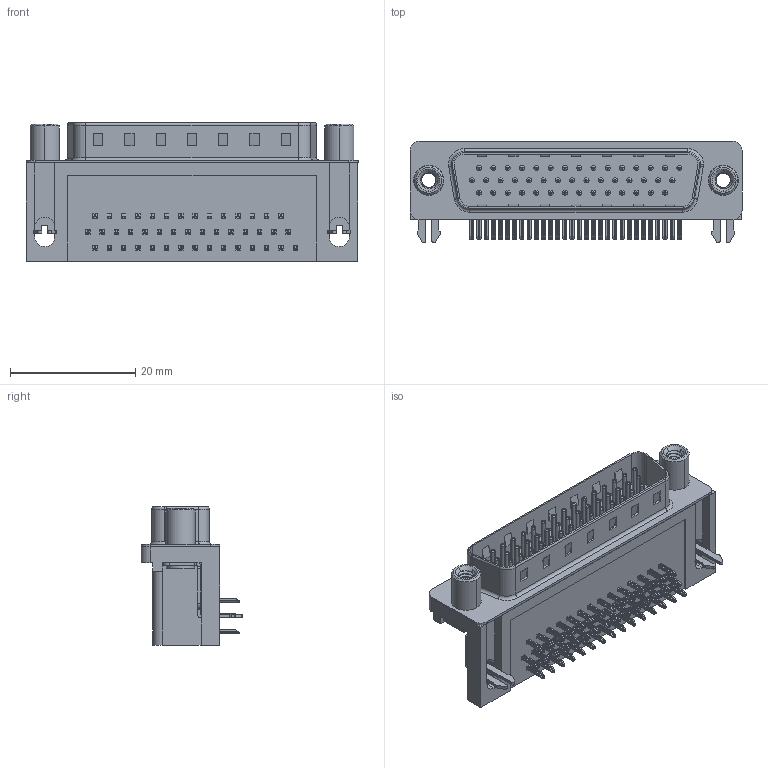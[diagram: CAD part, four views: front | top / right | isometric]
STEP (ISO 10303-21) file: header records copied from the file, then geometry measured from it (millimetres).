
FILE_DESCRIPTION (( 'STEP AP203' ), '1' );
FILE_NAME ('633-044-263-530.STEP', '2018-09-07T14:01:23', ( '' ), ( '' ), 'SwSTEP 2.0', 'SolidWorks 2016', '' );
FILE_SCHEMA (( 'CONFIG_CONTROL_DESIGN' ));
Length unit declared in the file: millimetre
Products named in the file (8): 633 Contact Middle; 633 Contact Top; 633 2 Prong Board Lock; 633 Round Threaded Standoff; 633-044-263-530; 633 Housing_44 Contact; 633 Shell_44 Contact; 633 Contact Bottom
Assembly tree (50 placements, depth 2):
  633-044-263-530
    633 Housing_44 Contact
    633 Shell_44 Contact
    633 Contact Bottom  x14
    633 Contact Middle  x15
    633 Contact Top  x15
    633 2 Prong Board Lock  x2
    633 Round Threaded Standoff  x2
Bounding box: 53.04 x 16.25 x 22.1 mm (x, y, z)
Volume: 8204.3 mm3; surface area: 10422.1 mm2
Topology: 50 solids, 50 shells, 3724 faces, 9212 edges, 5681 vertices
Faces by surface type: plane 2341, cylinder 1076, torus 279, bspline 16, cone 12
Entity records: 30312 total; most frequent: CARTESIAN_POINT 6557, DIRECTION 4576, ORIENTED_EDGE 4408, EDGE_CURVE 2204, VECTOR 1568, LINE 1568, AXIS2_PLACEMENT_3D 1504, VERTEX_POINT 1421
